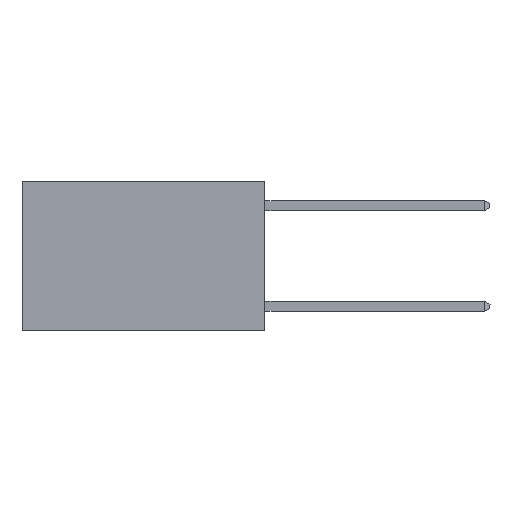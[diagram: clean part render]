
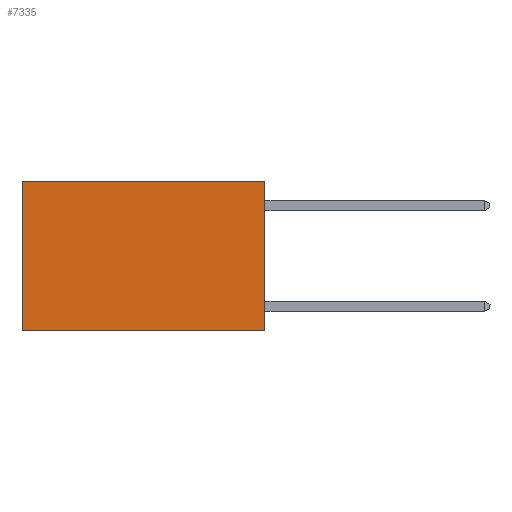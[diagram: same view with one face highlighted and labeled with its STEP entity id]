
A CAD part, left-side view. The second image highlights one B-rep face of the part: STEP entity #7335.
In plain terms, the highlighted planar face has unit normal (-1, 0, 0).
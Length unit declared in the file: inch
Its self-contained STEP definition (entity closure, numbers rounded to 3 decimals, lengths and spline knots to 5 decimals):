
#153 = VECTOR ( 'NONE', #2848, 39.37008 ) ;
#225 = VECTOR ( 'NONE', #2561, 39.37008 ) ;
#414 = DIRECTION ( 'NONE',  ( 0., 1., 0. ) ) ;
#720 = CARTESIAN_POINT ( 'NONE',  ( 0.2625, 0., 0. ) ) ;
#801 = CARTESIAN_POINT ( 'NONE',  ( 0.2625, 0., -0.37 ) ) ;
#2168 = LINE ( 'NONE', #801, #153 ) ;
#2278 = VECTOR ( 'NONE', #414, 39.37008 ) ;
#2333 = VERTEX_POINT ( 'NONE', #7341 ) ;
#2532 = CARTESIAN_POINT ( 'NONE',  ( 0.2625, 0.6, 0. ) ) ;
#2551 = VECTOR ( 'NONE', #6896, 39.37008 ) ;
#2561 = DIRECTION ( 'NONE',  ( 0., 0., -1. ) ) ;
#2563 = EDGE_CURVE ( 'NONE', #7355, #7358, #4329, .T. ) ;
#2664 = CARTESIAN_POINT ( 'NONE',  ( 0.2625, 0., 0. ) ) ;
#2787 = LINE ( 'NONE', #2664, #2551 ) ;
#2848 = DIRECTION ( 'NONE',  ( 0., 1., 0. ) ) ;
#2958 = VERTEX_POINT ( 'NONE', #4163 ) ;
#3395 = CARTESIAN_POINT ( 'NONE',  ( 0.2625, 0., 0. ) ) ;
#4070 = CARTESIAN_POINT ( 'NONE',  ( 0.2625, 0., 0. ) ) ;
#4163 = CARTESIAN_POINT ( 'NONE',  ( 0.2625, 0.6, -0.37 ) ) ;
#4198 = AXIS2_PLACEMENT_3D ( 'NONE', #4070, #6903, #5544 ) ;
#4329 = LINE ( 'NONE', #720, #2278 ) ;
#4595 = ORIENTED_EDGE ( 'NONE', *, *, #2563, .T. ) ;
#4806 = PLANE ( 'NONE',  #4198 ) ;
#5544 = DIRECTION ( 'NONE',  ( 0., 0., -1. ) ) ;
#5785 = LINE ( 'NONE', #2532, #225 ) ;
#6203 = EDGE_CURVE ( 'NONE', #2333, #2958, #2168, .T. ) ;
#6896 = DIRECTION ( 'NONE',  ( 0., 0., -1. ) ) ;
#6903 = DIRECTION ( 'NONE',  ( 1., 0., 0. ) ) ;
#7268 = EDGE_LOOP ( 'NONE', ( #7591, #8131, #8691, #4595 ) ) ;
#7335 = ADVANCED_FACE ( 'NONE', ( #8294 ), #4806, .F. ) ;
#7341 = CARTESIAN_POINT ( 'NONE',  ( 0.2625, 0., -0.37 ) ) ;
#7355 = VERTEX_POINT ( 'NONE', #3395 ) ;
#7358 = VERTEX_POINT ( 'NONE', #8230 ) ;
#7591 = ORIENTED_EDGE ( 'NONE', *, *, #8790, .T. ) ;
#8016 = EDGE_CURVE ( 'NONE', #7355, #2333, #2787, .T. ) ;
#8131 = ORIENTED_EDGE ( 'NONE', *, *, #6203, .F. ) ;
#8230 = CARTESIAN_POINT ( 'NONE',  ( 0.2625, 0.6, 0. ) ) ;
#8294 = FACE_OUTER_BOUND ( 'NONE', #7268, .T. ) ;
#8691 = ORIENTED_EDGE ( 'NONE', *, *, #8016, .F. ) ;
#8790 = EDGE_CURVE ( 'NONE', #7358, #2958, #5785, .T. ) ;
